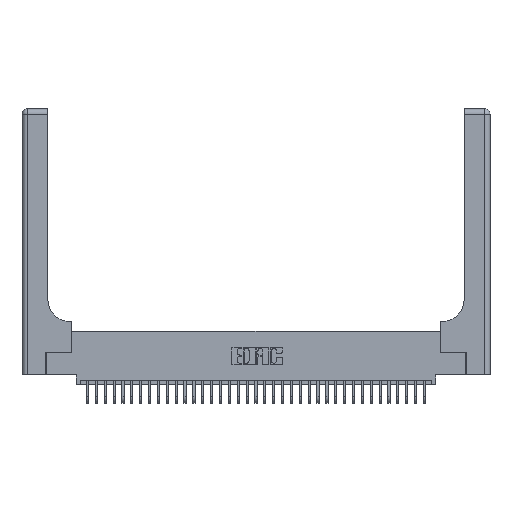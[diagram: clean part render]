
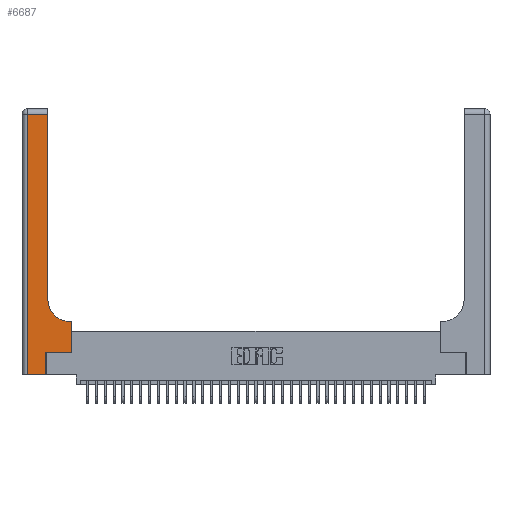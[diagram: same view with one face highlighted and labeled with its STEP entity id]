
A CAD part, top view. The second image highlights one B-rep face of the part: STEP entity #6687.
In plain terms, the highlighted planar face has unit normal (0, 0, 1).
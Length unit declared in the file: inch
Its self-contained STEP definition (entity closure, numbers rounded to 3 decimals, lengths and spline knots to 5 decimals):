
#14 = VERTEX_POINT ( 'NONE', #6575 ) ;
#1507 = ORIENTED_EDGE ( 'NONE', *, *, #17034, .T. ) ;
#1591 = EDGE_CURVE ( 'NONE', #25215, #14414, #8115, .T. ) ;
#2010 = LINE ( 'NONE', #36272, #2971 ) ;
#2056 = DIRECTION ( 'NONE',  ( 0., -1., 0. ) ) ;
#2971 = VECTOR ( 'NONE', #18982, 39.37008 ) ;
#3365 = DIRECTION ( 'NONE',  ( 0., 1., 0. ) ) ;
#4226 = CARTESIAN_POINT ( 'NONE',  ( 0.269, 0.25, 0.37 ) ) ;
#5517 = DIRECTION ( 'NONE',  ( -1., 0., 0. ) ) ;
#5812 = AXIS2_PLACEMENT_3D ( 'NONE', #11356, #14372, #34658 ) ;
#6019 = ORIENTED_EDGE ( 'NONE', *, *, #6602, .T. ) ;
#6356 = DIRECTION ( 'NONE',  ( 0., 1., 0. ) ) ;
#6575 = CARTESIAN_POINT ( 'NONE',  ( 0.5415, 0.6, 0.37 ) ) ;
#6602 = EDGE_CURVE ( 'NONE', #14414, #20951, #15288, .T. ) ;
#6687 = ADVANCED_FACE ( 'NONE', ( #28036 ), #28867, .F. ) ;
#6930 = CARTESIAN_POINT ( 'NONE',  ( 0.2915, 0.6, 0.37 ) ) ;
#8115 = LINE ( 'NONE', #23241, #28776 ) ;
#10160 = ORIENTED_EDGE ( 'NONE', *, *, #18622, .T. ) ;
#11356 = CARTESIAN_POINT ( 'NONE',  ( 0., 3., 0.37 ) ) ;
#13042 = EDGE_CURVE ( 'NONE', #14, #20570, #23932, .T. ) ;
#13507 = VECTOR ( 'NONE', #13662, 39.37008 ) ;
#13662 = DIRECTION ( 'NONE',  ( 0., 1., 0. ) ) ;
#14372 = DIRECTION ( 'NONE',  ( 0., 0., -1. ) ) ;
#14414 = VERTEX_POINT ( 'NONE', #18191 ) ;
#15061 = DIRECTION ( 'NONE',  ( 0., 0., -1. ) ) ;
#15288 = LINE ( 'NONE', #19890, #24001 ) ;
#16015 = CARTESIAN_POINT ( 'NONE',  ( 0.2915, 0.85, 0.37 ) ) ;
#16237 = CARTESIAN_POINT ( 'NONE',  ( 0.269, 0.25, 0.37 ) ) ;
#16602 = CARTESIAN_POINT ( 'NONE',  ( 0.5585, 0.6, 0.37 ) ) ;
#17034 = EDGE_CURVE ( 'NONE', #21989, #19415, #28122, .T. ) ;
#17642 = CARTESIAN_POINT ( 'NONE',  ( 0.2915, 2.94, 0.37 ) ) ;
#17780 = ORIENTED_EDGE ( 'NONE', *, *, #36223, .T. ) ;
#17970 = ORIENTED_EDGE ( 'NONE', *, *, #35233, .T. ) ;
#18191 = CARTESIAN_POINT ( 'NONE',  ( 0.06, 2.94, 0.37 ) ) ;
#18622 = EDGE_CURVE ( 'NONE', #20951, #21989, #2010, .T. ) ;
#18782 = CARTESIAN_POINT ( 'NONE',  ( 0.269, 0., 0.37 ) ) ;
#18982 = DIRECTION ( 'NONE',  ( 1., 0., 0. ) ) ;
#19025 = CARTESIAN_POINT ( 'NONE',  ( 0.5585, 0.25, 0.37 ) ) ;
#19415 = VERTEX_POINT ( 'NONE', #16237 ) ;
#19890 = CARTESIAN_POINT ( 'NONE',  ( 0.06, 3., 0.37 ) ) ;
#20570 = VERTEX_POINT ( 'NONE', #16015 ) ;
#20951 = VERTEX_POINT ( 'NONE', #34874 ) ;
#21131 = CARTESIAN_POINT ( 'NONE',  ( 0.2915, 3., 0.37 ) ) ;
#21668 = DIRECTION ( 'NONE',  ( -1., 0., 0. ) ) ;
#21914 = VECTOR ( 'NONE', #3365, 39.37008 ) ;
#21989 = VERTEX_POINT ( 'NONE', #18782 ) ;
#21990 = DIRECTION ( 'NONE',  ( 1., 0., 0. ) ) ;
#22854 = LINE ( 'NONE', #21131, #21914 ) ;
#23241 = CARTESIAN_POINT ( 'NONE',  ( 0., 2.94, 0.37 ) ) ;
#23932 = CIRCLE ( 'NONE', #35111, 0.25 ) ;
#24001 = VECTOR ( 'NONE', #2056, 39.37008 ) ;
#24302 = VECTOR ( 'NONE', #6356, 39.37008 ) ;
#24639 = EDGE_CURVE ( 'NONE', #20570, #25215, #22854, .T. ) ;
#25092 = ORIENTED_EDGE ( 'NONE', *, *, #13042, .T. ) ;
#25215 = VERTEX_POINT ( 'NONE', #17642 ) ;
#25357 = ORIENTED_EDGE ( 'NONE', *, *, #1591, .T. ) ;
#26109 = EDGE_CURVE ( 'NONE', #35520, #14, #34467, .T. ) ;
#28036 = FACE_OUTER_BOUND ( 'NONE', #36383, .T. ) ;
#28122 = LINE ( 'NONE', #36889, #13507 ) ;
#28776 = VECTOR ( 'NONE', #5517, 39.37008 ) ;
#28867 = PLANE ( 'NONE',  #5812 ) ;
#29176 = VECTOR ( 'NONE', #21990, 39.37008 ) ;
#29722 = CARTESIAN_POINT ( 'NONE',  ( 0.5585, 0.25, 0.37 ) ) ;
#30601 = ORIENTED_EDGE ( 'NONE', *, *, #24639, .T. ) ;
#31974 = LINE ( 'NONE', #29722, #24302 ) ;
#32034 = ORIENTED_EDGE ( 'NONE', *, *, #26109, .T. ) ;
#32460 = CARTESIAN_POINT ( 'NONE',  ( 0.5415, 0.85, 0.37 ) ) ;
#33568 = VECTOR ( 'NONE', #21668, 39.37008 ) ;
#34467 = LINE ( 'NONE', #6930, #33568 ) ;
#34658 = DIRECTION ( 'NONE',  ( -1., 0., 0. ) ) ;
#34874 = CARTESIAN_POINT ( 'NONE',  ( 0.06, 0., 0.37 ) ) ;
#35111 = AXIS2_PLACEMENT_3D ( 'NONE', #32460, #15061, #35348 ) ;
#35233 = EDGE_CURVE ( 'NONE', #36848, #35520, #31974, .T. ) ;
#35348 = DIRECTION ( 'NONE',  ( 1., 0., 0. ) ) ;
#35520 = VERTEX_POINT ( 'NONE', #16602 ) ;
#36223 = EDGE_CURVE ( 'NONE', #19415, #36848, #37741, .T. ) ;
#36272 = CARTESIAN_POINT ( 'NONE',  ( 0., 0., 0.37 ) ) ;
#36383 = EDGE_LOOP ( 'NONE', ( #30601, #25357, #6019, #10160, #1507, #17780, #17970, #32034, #25092 ) ) ;
#36848 = VERTEX_POINT ( 'NONE', #19025 ) ;
#36889 = CARTESIAN_POINT ( 'NONE',  ( 0.269, 0., 0.37 ) ) ;
#37741 = LINE ( 'NONE', #4226, #29176 ) ;
